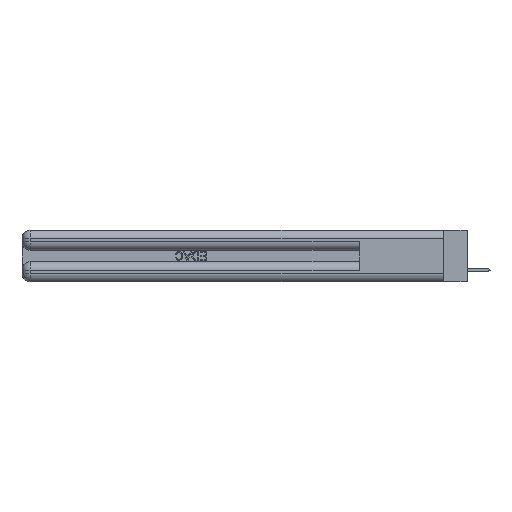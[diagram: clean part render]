
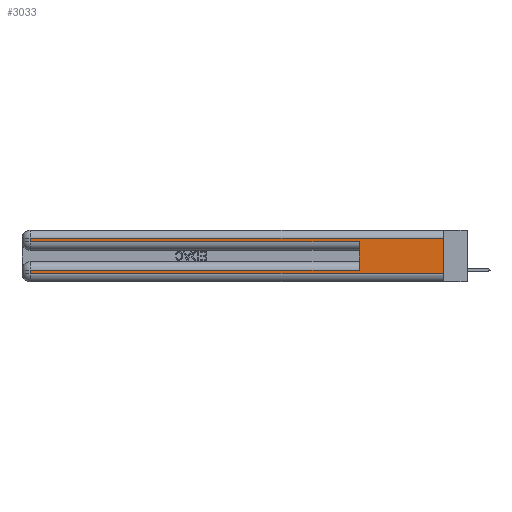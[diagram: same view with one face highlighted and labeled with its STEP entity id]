
A CAD part, left-side view. The second image highlights one B-rep face of the part: STEP entity #3033.
In plain terms, the highlighted planar face has unit normal (-1, 0, 0).
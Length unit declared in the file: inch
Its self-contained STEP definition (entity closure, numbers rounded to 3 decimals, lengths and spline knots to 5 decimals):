
#263 = EDGE_LOOP ( 'NONE', ( #28672, #34127, #34981, #30780, #22429, #43478, #22123, #24036 ) ) ;
#1353 = LINE ( 'NONE', #6594, #17357 ) ;
#1621 = VERTEX_POINT ( 'NONE', #24231 ) ;
#2571 = DIRECTION ( 'NONE',  ( 0., 0., 1. ) ) ;
#3033 = ADVANCED_FACE ( 'NONE', ( #24355 ), #12968, .F. ) ;
#4597 = EDGE_CURVE ( 'NONE', #42750, #35389, #1353, .T. ) ;
#5110 = CARTESIAN_POINT ( 'NONE',  ( 0., 2.94, 0.085 ) ) ;
#6194 = DIRECTION ( 'NONE',  ( 0., -1., 0. ) ) ;
#6261 = VECTOR ( 'NONE', #44638, 39.37008 ) ;
#6594 = CARTESIAN_POINT ( 'NONE',  ( 0., 0.6, 0.145 ) ) ;
#8086 = EDGE_CURVE ( 'NONE', #34330, #35389, #10533, .T. ) ;
#8220 = EDGE_CURVE ( 'NONE', #1621, #20969, #33927, .T. ) ;
#9262 = CARTESIAN_POINT ( 'NONE',  ( 0., 2.94, 0.285 ) ) ;
#9394 = VECTOR ( 'NONE', #41620, 39.37008 ) ;
#10477 = DIRECTION ( 'NONE',  ( 0., 0., -1. ) ) ;
#10484 = EDGE_CURVE ( 'NONE', #1621, #11738, #15960, .T. ) ;
#10533 = LINE ( 'NONE', #15941, #9394 ) ;
#10872 = DIRECTION ( 'NONE',  ( 0., 0., -1. ) ) ;
#11332 = LINE ( 'NONE', #21182, #27918 ) ;
#11738 = VERTEX_POINT ( 'NONE', #17165 ) ;
#12655 = DIRECTION ( 'NONE',  ( 0., 0., -1. ) ) ;
#12968 = PLANE ( 'NONE',  #24486 ) ;
#13532 = DIRECTION ( 'NONE',  ( 0., 0., -1. ) ) ;
#13982 = CARTESIAN_POINT ( 'NONE',  ( 0., 0., 0.085 ) ) ;
#14034 = LINE ( 'NONE', #25466, #30643 ) ;
#15875 = CARTESIAN_POINT ( 'NONE',  ( 0., 2.94, 0.06 ) ) ;
#15941 = CARTESIAN_POINT ( 'NONE',  ( 0., 0., 0.285 ) ) ;
#15960 = LINE ( 'NONE', #41479, #6261 ) ;
#16859 = VECTOR ( 'NONE', #39954, 39.37008 ) ;
#17165 = CARTESIAN_POINT ( 'NONE',  ( 0., 2.94, 0.31 ) ) ;
#17357 = VECTOR ( 'NONE', #2571, 39.37008 ) ;
#19826 = CARTESIAN_POINT ( 'NONE',  ( 0., 0., 0.37 ) ) ;
#20969 = VERTEX_POINT ( 'NONE', #43595 ) ;
#21182 = CARTESIAN_POINT ( 'NONE',  ( 0., 0., 0.06 ) ) ;
#21388 = CARTESIAN_POINT ( 'NONE',  ( 0., 2.94, 0.37 ) ) ;
#22123 = ORIENTED_EDGE ( 'NONE', *, *, #38859, .T. ) ;
#22429 = ORIENTED_EDGE ( 'NONE', *, *, #4597, .F. ) ;
#23075 = VECTOR ( 'NONE', #10872, 39.37008 ) ;
#24036 = ORIENTED_EDGE ( 'NONE', *, *, #35879, .T. ) ;
#24231 = CARTESIAN_POINT ( 'NONE',  ( 0., 0., 0.31 ) ) ;
#24355 = FACE_OUTER_BOUND ( 'NONE', #263, .T. ) ;
#24486 = AXIS2_PLACEMENT_3D ( 'NONE', #19826, #30882, #12655 ) ;
#25466 = CARTESIAN_POINT ( 'NONE',  ( 0., 2.94, 0.37 ) ) ;
#27102 = LINE ( 'NONE', #21388, #23075 ) ;
#27918 = VECTOR ( 'NONE', #6194, 39.37008 ) ;
#28672 = ORIENTED_EDGE ( 'NONE', *, *, #8220, .F. ) ;
#29549 = CARTESIAN_POINT ( 'NONE',  ( 0., 0.6, 0.285 ) ) ;
#30643 = VECTOR ( 'NONE', #10477, 39.37008 ) ;
#30780 = ORIENTED_EDGE ( 'NONE', *, *, #8086, .T. ) ;
#30882 = DIRECTION ( 'NONE',  ( 1., 0., 0. ) ) ;
#33927 = LINE ( 'NONE', #46067, #41427 ) ;
#34127 = ORIENTED_EDGE ( 'NONE', *, *, #10484, .T. ) ;
#34330 = VERTEX_POINT ( 'NONE', #9262 ) ;
#34687 = LINE ( 'NONE', #13982, #16859 ) ;
#34981 = ORIENTED_EDGE ( 'NONE', *, *, #47083, .T. ) ;
#35389 = VERTEX_POINT ( 'NONE', #29549 ) ;
#35623 = VERTEX_POINT ( 'NONE', #5110 ) ;
#35879 = EDGE_CURVE ( 'NONE', #43003, #20969, #11332, .T. ) ;
#37673 = EDGE_CURVE ( 'NONE', #42750, #35623, #34687, .T. ) ;
#38859 = EDGE_CURVE ( 'NONE', #35623, #43003, #27102, .T. ) ;
#39954 = DIRECTION ( 'NONE',  ( 0., 1., 0. ) ) ;
#41427 = VECTOR ( 'NONE', #13532, 39.37008 ) ;
#41479 = CARTESIAN_POINT ( 'NONE',  ( 0., 0., 0.31 ) ) ;
#41620 = DIRECTION ( 'NONE',  ( 0., -1., 0. ) ) ;
#42750 = VERTEX_POINT ( 'NONE', #46294 ) ;
#43003 = VERTEX_POINT ( 'NONE', #15875 ) ;
#43478 = ORIENTED_EDGE ( 'NONE', *, *, #37673, .T. ) ;
#43595 = CARTESIAN_POINT ( 'NONE',  ( 0., 0., 0.06 ) ) ;
#44638 = DIRECTION ( 'NONE',  ( 0., 1., 0. ) ) ;
#46067 = CARTESIAN_POINT ( 'NONE',  ( 0., 0., 0.37 ) ) ;
#46294 = CARTESIAN_POINT ( 'NONE',  ( 0., 0.6, 0.085 ) ) ;
#47083 = EDGE_CURVE ( 'NONE', #11738, #34330, #14034, .T. ) ;
